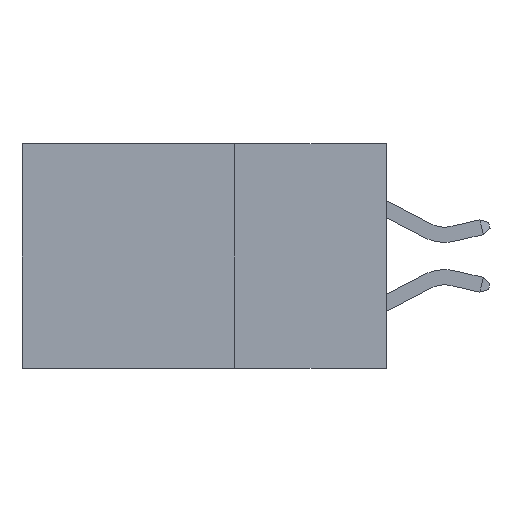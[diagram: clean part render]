
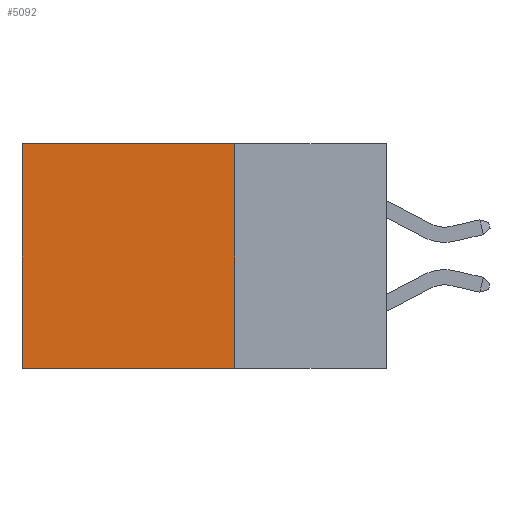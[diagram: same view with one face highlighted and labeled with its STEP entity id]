
A CAD part, left-side view. The second image highlights one B-rep face of the part: STEP entity #5092.
In plain terms, the highlighted planar face has unit normal (-1, 0, 0).
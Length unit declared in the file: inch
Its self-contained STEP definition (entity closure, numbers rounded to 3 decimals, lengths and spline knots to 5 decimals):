
#239 = VERTEX_POINT ( 'NONE', #16982 ) ;
#855 = VERTEX_POINT ( 'NONE', #15974 ) ;
#1818 = LINE ( 'NONE', #11672, #14861 ) ;
#3398 = VECTOR ( 'NONE', #15511, 39.37008 ) ;
#4620 = LINE ( 'NONE', #11297, #12135 ) ;
#4725 = DIRECTION ( 'NONE',  ( 0., 0., -1. ) ) ;
#5092 = ADVANCED_FACE ( 'NONE', ( #14089 ), #10726, .F. ) ;
#5567 = EDGE_CURVE ( 'NONE', #20643, #855, #19312, .T. ) ;
#5660 = CARTESIAN_POINT ( 'NONE',  ( 0.2615, 0.25, 0. ) ) ;
#6080 = DIRECTION ( 'NONE',  ( 0., 1., 0. ) ) ;
#6627 = ORIENTED_EDGE ( 'NONE', *, *, #9224, .T. ) ;
#6979 = DIRECTION ( 'NONE',  ( 0., 0., -1. ) ) ;
#7726 = CARTESIAN_POINT ( 'NONE',  ( 0.2615, 0.25, -0.37 ) ) ;
#8095 = AXIS2_PLACEMENT_3D ( 'NONE', #12577, #19033, #14208 ) ;
#9224 = EDGE_CURVE ( 'NONE', #239, #855, #1818, .T. ) ;
#10589 = LINE ( 'NONE', #5660, #3398 ) ;
#10726 = PLANE ( 'NONE',  #8095 ) ;
#11297 = CARTESIAN_POINT ( 'NONE',  ( 0.2615, 0.25, -0.37 ) ) ;
#11672 = CARTESIAN_POINT ( 'NONE',  ( 0.2615, 0.6, -0.37 ) ) ;
#11772 = ORIENTED_EDGE ( 'NONE', *, *, #5567, .F. ) ;
#12135 = VECTOR ( 'NONE', #4725, 39.37008 ) ;
#12577 = CARTESIAN_POINT ( 'NONE',  ( 0.2615, 0.25, -0.37 ) ) ;
#12847 = VERTEX_POINT ( 'NONE', #15654 ) ;
#13533 = EDGE_CURVE ( 'NONE', #12847, #20643, #4620, .T. ) ;
#14089 = FACE_OUTER_BOUND ( 'NONE', #19161, .T. ) ;
#14208 = DIRECTION ( 'NONE',  ( 0., 0., -1. ) ) ;
#14861 = VECTOR ( 'NONE', #6979, 39.37008 ) ;
#15511 = DIRECTION ( 'NONE',  ( 0., 1., 0. ) ) ;
#15654 = CARTESIAN_POINT ( 'NONE',  ( 0.2615, 0.25, 0. ) ) ;
#15808 = ORIENTED_EDGE ( 'NONE', *, *, #13533, .F. ) ;
#15974 = CARTESIAN_POINT ( 'NONE',  ( 0.2615, 0.6, -0.37 ) ) ;
#16547 = ORIENTED_EDGE ( 'NONE', *, *, #19474, .T. ) ;
#16982 = CARTESIAN_POINT ( 'NONE',  ( 0.2615, 0.6, 0. ) ) ;
#17596 = CARTESIAN_POINT ( 'NONE',  ( 0.2615, 0.25, -0.37 ) ) ;
#19033 = DIRECTION ( 'NONE',  ( 1., 0., 0. ) ) ;
#19161 = EDGE_LOOP ( 'NONE', ( #6627, #11772, #15808, #16547 ) ) ;
#19312 = LINE ( 'NONE', #7726, #20706 ) ;
#19474 = EDGE_CURVE ( 'NONE', #12847, #239, #10589, .T. ) ;
#20643 = VERTEX_POINT ( 'NONE', #17596 ) ;
#20706 = VECTOR ( 'NONE', #6080, 39.37008 ) ;
